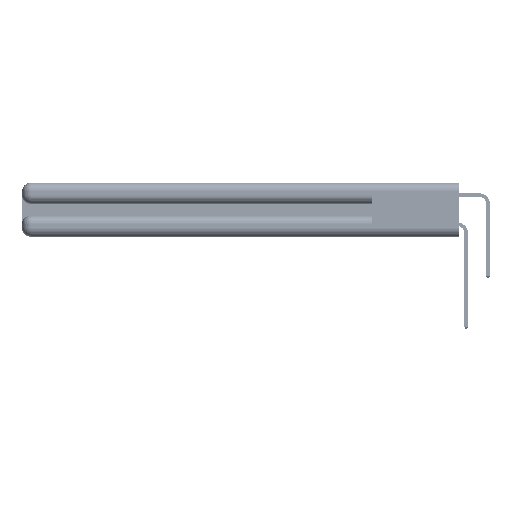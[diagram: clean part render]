
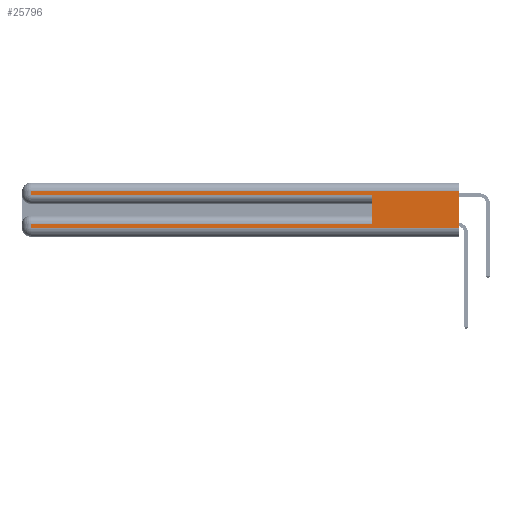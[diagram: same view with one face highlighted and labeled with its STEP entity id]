
A CAD part, left-side view. The second image highlights one B-rep face of the part: STEP entity #25796.
In plain terms, the highlighted planar face has unit normal (-1, 0, 0).
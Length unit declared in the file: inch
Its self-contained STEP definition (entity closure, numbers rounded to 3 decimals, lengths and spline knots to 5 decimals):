
#1617 = PLANE ( 'NONE',  #44942 ) ;
#1630 = CARTESIAN_POINT ( 'NONE',  ( 0., 0., 0.37 ) ) ;
#2779 = CARTESIAN_POINT ( 'NONE',  ( 0., 0.6, 0.285 ) ) ;
#4336 = LINE ( 'NONE', #45476, #34793 ) ;
#4995 = VERTEX_POINT ( 'NONE', #2779 ) ;
#5629 = CARTESIAN_POINT ( 'NONE',  ( 0., 0., 0.37 ) ) ;
#7966 = CARTESIAN_POINT ( 'NONE',  ( 0., 2.94, 0.285 ) ) ;
#9626 = DIRECTION ( 'NONE',  ( 1., 0., 0. ) ) ;
#9636 = DIRECTION ( 'NONE',  ( 0., 0., -1. ) ) ;
#9756 = CARTESIAN_POINT ( 'NONE',  ( 0., 0.6, 0.145 ) ) ;
#10224 = CARTESIAN_POINT ( 'NONE',  ( 0., 2.94, 0.37 ) ) ;
#10234 = VECTOR ( 'NONE', #47522, 39.37008 ) ;
#11838 = EDGE_CURVE ( 'NONE', #40993, #37489, #29428, .T. ) ;
#12935 = VERTEX_POINT ( 'NONE', #51458 ) ;
#13028 = EDGE_CURVE ( 'NONE', #12935, #43517, #36735, .T. ) ;
#14691 = LINE ( 'NONE', #47954, #35810 ) ;
#15052 = ORIENTED_EDGE ( 'NONE', *, *, #11838, .T. ) ;
#15079 = VERTEX_POINT ( 'NONE', #26385 ) ;
#15382 = EDGE_LOOP ( 'NONE', ( #26374, #35786, #15052, #39256, #20087, #48558, #29425, #49352 ) ) ;
#15601 = VECTOR ( 'NONE', #48133, 39.37008 ) ;
#17479 = EDGE_CURVE ( 'NONE', #28178, #43517, #36022, .T. ) ;
#18098 = EDGE_CURVE ( 'NONE', #31482, #4995, #37848, .T. ) ;
#19017 = DIRECTION ( 'NONE',  ( 0., -1., 0. ) ) ;
#19734 = CARTESIAN_POINT ( 'NONE',  ( 0., 2.94, 0.37 ) ) ;
#19877 = CARTESIAN_POINT ( 'NONE',  ( 0., 2.94, 0.31 ) ) ;
#20087 = ORIENTED_EDGE ( 'NONE', *, *, #18098, .F. ) ;
#20168 = DIRECTION ( 'NONE',  ( 0., 1., 0. ) ) ;
#20932 = LINE ( 'NONE', #38827, #50117 ) ;
#22230 = DIRECTION ( 'NONE',  ( 0., 0., -1. ) ) ;
#22977 = VECTOR ( 'NONE', #9636, 39.37008 ) ;
#23944 = EDGE_CURVE ( 'NONE', #37489, #4995, #20932, .T. ) ;
#25796 = ADVANCED_FACE ( 'NONE', ( #51173 ), #1617, .F. ) ;
#26374 = ORIENTED_EDGE ( 'NONE', *, *, #17479, .F. ) ;
#26385 = CARTESIAN_POINT ( 'NONE',  ( 0., 2.94, 0.085 ) ) ;
#27190 = CARTESIAN_POINT ( 'NONE',  ( 0., 0., 0.31 ) ) ;
#27538 = EDGE_CURVE ( 'NONE', #31482, #15079, #4336, .T. ) ;
#28178 = VERTEX_POINT ( 'NONE', #27190 ) ;
#29057 = EDGE_CURVE ( 'NONE', #28178, #40993, #14691, .T. ) ;
#29425 = ORIENTED_EDGE ( 'NONE', *, *, #43493, .T. ) ;
#29428 = LINE ( 'NONE', #10224, #39994 ) ;
#31482 = VERTEX_POINT ( 'NONE', #41674 ) ;
#34793 = VECTOR ( 'NONE', #50524, 39.37008 ) ;
#35786 = ORIENTED_EDGE ( 'NONE', *, *, #29057, .T. ) ;
#35810 = VECTOR ( 'NONE', #20168, 39.37008 ) ;
#36022 = LINE ( 'NONE', #1630, #22977 ) ;
#36579 = VECTOR ( 'NONE', #41571, 39.37008 ) ;
#36735 = LINE ( 'NONE', #44132, #15601 ) ;
#37451 = DIRECTION ( 'NONE',  ( 0., 0., -1. ) ) ;
#37489 = VERTEX_POINT ( 'NONE', #7966 ) ;
#37848 = LINE ( 'NONE', #9756, #36579 ) ;
#38827 = CARTESIAN_POINT ( 'NONE',  ( 0., 0., 0.285 ) ) ;
#39256 = ORIENTED_EDGE ( 'NONE', *, *, #23944, .T. ) ;
#39994 = VECTOR ( 'NONE', #22230, 39.37008 ) ;
#40993 = VERTEX_POINT ( 'NONE', #19877 ) ;
#41571 = DIRECTION ( 'NONE',  ( 0., 0., 1. ) ) ;
#41674 = CARTESIAN_POINT ( 'NONE',  ( 0., 0.6, 0.085 ) ) ;
#43493 = EDGE_CURVE ( 'NONE', #15079, #12935, #51282, .T. ) ;
#43517 = VERTEX_POINT ( 'NONE', #44972 ) ;
#44132 = CARTESIAN_POINT ( 'NONE',  ( 0., 0., 0.06 ) ) ;
#44942 = AXIS2_PLACEMENT_3D ( 'NONE', #5629, #9626, #37451 ) ;
#44972 = CARTESIAN_POINT ( 'NONE',  ( 0., 0., 0.06 ) ) ;
#45476 = CARTESIAN_POINT ( 'NONE',  ( 0., 0., 0.085 ) ) ;
#47522 = DIRECTION ( 'NONE',  ( 0., 0., -1. ) ) ;
#47954 = CARTESIAN_POINT ( 'NONE',  ( 0., 0., 0.31 ) ) ;
#48133 = DIRECTION ( 'NONE',  ( 0., -1., 0. ) ) ;
#48558 = ORIENTED_EDGE ( 'NONE', *, *, #27538, .T. ) ;
#49352 = ORIENTED_EDGE ( 'NONE', *, *, #13028, .T. ) ;
#50117 = VECTOR ( 'NONE', #19017, 39.37008 ) ;
#50524 = DIRECTION ( 'NONE',  ( 0., 1., 0. ) ) ;
#51173 = FACE_OUTER_BOUND ( 'NONE', #15382, .T. ) ;
#51282 = LINE ( 'NONE', #19734, #10234 ) ;
#51458 = CARTESIAN_POINT ( 'NONE',  ( 0., 2.94, 0.06 ) ) ;
